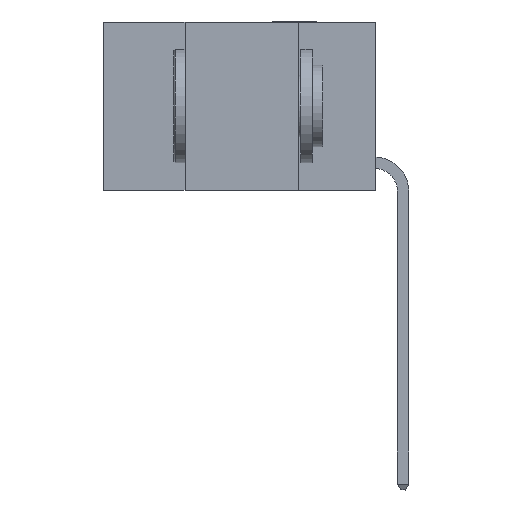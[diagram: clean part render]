
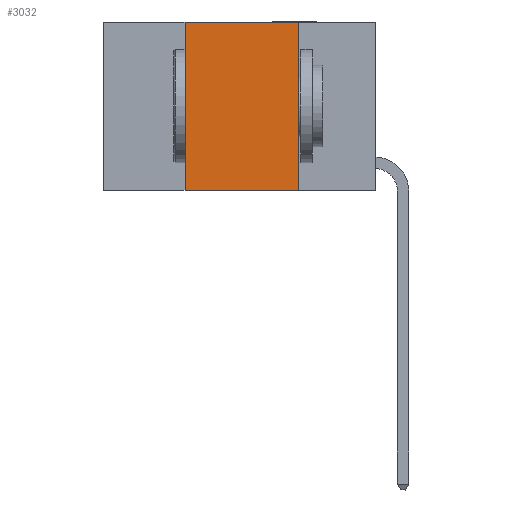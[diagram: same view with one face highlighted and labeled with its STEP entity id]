
A CAD part, left-side view. The second image highlights one B-rep face of the part: STEP entity #3032.
In plain terms, the highlighted planar face has unit normal (-1, 0, 0).
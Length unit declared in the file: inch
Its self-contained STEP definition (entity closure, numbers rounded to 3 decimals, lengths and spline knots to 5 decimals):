
#42 = ORIENTED_EDGE ( 'NONE', *, *, #8482, .T. ) ;
#224 = DIRECTION ( 'NONE',  ( 0., 0., -1. ) ) ;
#405 = CARTESIAN_POINT ( 'NONE',  ( 0., 0.6, 0. ) ) ;
#751 = EDGE_CURVE ( 'NONE', #9167, #4998, #6981, .T. ) ;
#857 = VECTOR ( 'NONE', #4489, 39.37008 ) ;
#1327 = EDGE_LOOP ( 'NONE', ( #6880, #1893, #2037, #42 ) ) ;
#1494 = VECTOR ( 'NONE', #3261, 39.37008 ) ;
#1846 = CARTESIAN_POINT ( 'NONE',  ( 0., 0.42, 0. ) ) ;
#1893 = ORIENTED_EDGE ( 'NONE', *, *, #8943, .F. ) ;
#2037 = ORIENTED_EDGE ( 'NONE', *, *, #5880, .F. ) ;
#2466 = CARTESIAN_POINT ( 'NONE',  ( 0., 0.42, 0. ) ) ;
#2788 = CARTESIAN_POINT ( 'NONE',  ( 0., 0.42, -0.37 ) ) ;
#3032 = ADVANCED_FACE ( 'NONE', ( #5862 ), #3467, .F. ) ;
#3261 = DIRECTION ( 'NONE',  ( 0., 0., 1. ) ) ;
#3467 = PLANE ( 'NONE',  #8539 ) ;
#4489 = DIRECTION ( 'NONE',  ( 0., -1., 0. ) ) ;
#4938 = VECTOR ( 'NONE', #9520, 39.37008 ) ;
#4998 = VERTEX_POINT ( 'NONE', #8663 ) ;
#5116 = DIRECTION ( 'NONE',  ( 1., 0., 0. ) ) ;
#5181 = LINE ( 'NONE', #405, #857 ) ;
#5862 = FACE_OUTER_BOUND ( 'NONE', #1327, .T. ) ;
#5880 = EDGE_CURVE ( 'NONE', #6222, #7352, #8429, .T. ) ;
#6222 = VERTEX_POINT ( 'NONE', #2788 ) ;
#6880 = ORIENTED_EDGE ( 'NONE', *, *, #751, .F. ) ;
#6981 = LINE ( 'NONE', #9942, #7226 ) ;
#7103 = LINE ( 'NONE', #8744, #4938 ) ;
#7178 = CARTESIAN_POINT ( 'NONE',  ( 0., 0.17, 0. ) ) ;
#7226 = VECTOR ( 'NONE', #9747, 39.37008 ) ;
#7352 = VERTEX_POINT ( 'NONE', #1846 ) ;
#8429 = LINE ( 'NONE', #2466, #1494 ) ;
#8482 = EDGE_CURVE ( 'NONE', #6222, #4998, #7103, .T. ) ;
#8539 = AXIS2_PLACEMENT_3D ( 'NONE', #9859, #5116, #224 ) ;
#8663 = CARTESIAN_POINT ( 'NONE',  ( 0., 0.17, -0.37 ) ) ;
#8744 = CARTESIAN_POINT ( 'NONE',  ( 0., 0.6, -0.37 ) ) ;
#8943 = EDGE_CURVE ( 'NONE', #7352, #9167, #5181, .T. ) ;
#9167 = VERTEX_POINT ( 'NONE', #7178 ) ;
#9520 = DIRECTION ( 'NONE',  ( 0., -1., 0. ) ) ;
#9747 = DIRECTION ( 'NONE',  ( 0., 0., -1. ) ) ;
#9859 = CARTESIAN_POINT ( 'NONE',  ( 0., 0.6, 0. ) ) ;
#9942 = CARTESIAN_POINT ( 'NONE',  ( 0., 0.17, 0. ) ) ;
